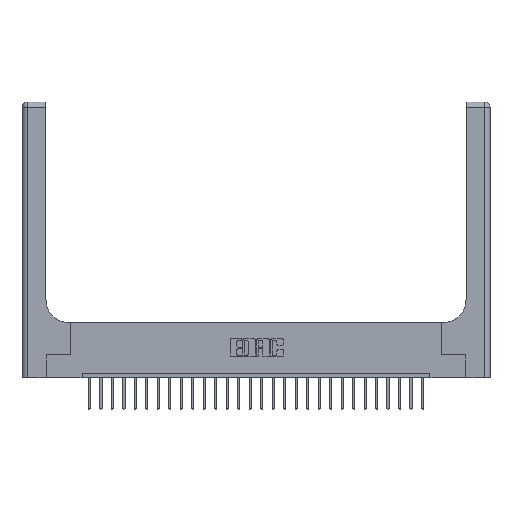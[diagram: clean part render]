
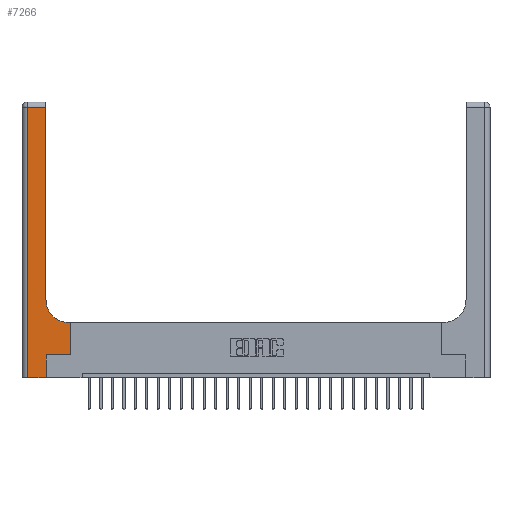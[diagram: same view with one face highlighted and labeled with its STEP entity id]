
A CAD part, top view. The second image highlights one B-rep face of the part: STEP entity #7266.
In plain terms, the highlighted planar face has unit normal (0, 0, 1).
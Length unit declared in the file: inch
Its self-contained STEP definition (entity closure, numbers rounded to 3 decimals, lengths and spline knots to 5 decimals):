
#961 = DIRECTION ( 'NONE',  ( 0., 1., 0. ) ) ;
#1334 = VECTOR ( 'NONE', #24281, 39.37008 ) ;
#1425 = EDGE_CURVE ( 'NONE', #2636, #16822, #12654, .T. ) ;
#1494 = DIRECTION ( 'NONE',  ( -1., 0., 0. ) ) ;
#1796 = CARTESIAN_POINT ( 'NONE',  ( 0.528, 0.6, 0.37 ) ) ;
#2108 = CARTESIAN_POINT ( 'NONE',  ( 0.265, 0., 0.37 ) ) ;
#2231 = CARTESIAN_POINT ( 'NONE',  ( 0., 0., 0.37 ) ) ;
#2236 = CARTESIAN_POINT ( 'NONE',  ( 0.26, 0.85, 0.37 ) ) ;
#2301 = VECTOR ( 'NONE', #20132, 39.37008 ) ;
#2636 = VERTEX_POINT ( 'NONE', #6936 ) ;
#2758 = VECTOR ( 'NONE', #10732, 39.37008 ) ;
#2800 = CARTESIAN_POINT ( 'NONE',  ( 0.06, 0., 0.37 ) ) ;
#2827 = CARTESIAN_POINT ( 'NONE',  ( 0.51, 0.6, 0.37 ) ) ;
#2962 = CARTESIAN_POINT ( 'NONE',  ( 0.528, 0.25, 0.37 ) ) ;
#3476 = CARTESIAN_POINT ( 'NONE',  ( 0., 3., 0.37 ) ) ;
#4074 = EDGE_CURVE ( 'NONE', #16822, #13934, #15352, .T. ) ;
#5895 = DIRECTION ( 'NONE',  ( -1., 0., 0. ) ) ;
#6661 = VERTEX_POINT ( 'NONE', #17787 ) ;
#6698 = VERTEX_POINT ( 'NONE', #2108 ) ;
#6707 = LINE ( 'NONE', #2231, #15286 ) ;
#6883 = CARTESIAN_POINT ( 'NONE',  ( 0.265, 0., 0.37 ) ) ;
#6888 = EDGE_CURVE ( 'NONE', #24734, #6661, #19367, .T. ) ;
#6936 = CARTESIAN_POINT ( 'NONE',  ( 0.265, 0.25, 0.37 ) ) ;
#7266 = ADVANCED_FACE ( 'NONE', ( #25118 ), #19017, .F. ) ;
#7838 = ORIENTED_EDGE ( 'NONE', *, *, #13670, .T. ) ;
#8047 = AXIS2_PLACEMENT_3D ( 'NONE', #11164, #24943, #13139 ) ;
#8358 = VERTEX_POINT ( 'NONE', #2236 ) ;
#8933 = EDGE_CURVE ( 'NONE', #13934, #12907, #24109, .T. ) ;
#9384 = ORIENTED_EDGE ( 'NONE', *, *, #17125, .T. ) ;
#9866 = ORIENTED_EDGE ( 'NONE', *, *, #15569, .T. ) ;
#10262 = CARTESIAN_POINT ( 'NONE',  ( 0.26, 3., 0.37 ) ) ;
#10732 = DIRECTION ( 'NONE',  ( 0., 1., 0. ) ) ;
#11164 = CARTESIAN_POINT ( 'NONE',  ( 0.51, 0.85, 0.37 ) ) ;
#11544 = DIRECTION ( 'NONE',  ( 1., 0., 0. ) ) ;
#11683 = ORIENTED_EDGE ( 'NONE', *, *, #1425, .T. ) ;
#12654 = LINE ( 'NONE', #21332, #20659 ) ;
#12907 = VERTEX_POINT ( 'NONE', #2827 ) ;
#13139 = DIRECTION ( 'NONE',  ( 1., 0., 0. ) ) ;
#13670 = EDGE_CURVE ( 'NONE', #23926, #6698, #6707, .T. ) ;
#13934 = VERTEX_POINT ( 'NONE', #1796 ) ;
#13953 = CARTESIAN_POINT ( 'NONE',  ( 0.26, 0.6, 0.37 ) ) ;
#14680 = ORIENTED_EDGE ( 'NONE', *, *, #4074, .T. ) ;
#15101 = CARTESIAN_POINT ( 'NONE',  ( 0.528, 0.25, 0.37 ) ) ;
#15286 = VECTOR ( 'NONE', #17718, 39.37008 ) ;
#15352 = LINE ( 'NONE', #2962, #2758 ) ;
#15569 = EDGE_CURVE ( 'NONE', #6661, #23926, #19903, .T. ) ;
#15830 = LINE ( 'NONE', #6883, #19542 ) ;
#16517 = AXIS2_PLACEMENT_3D ( 'NONE', #3476, #22923, #1494 ) ;
#16822 = VERTEX_POINT ( 'NONE', #15101 ) ;
#17125 = EDGE_CURVE ( 'NONE', #6698, #2636, #15830, .T. ) ;
#17254 = VECTOR ( 'NONE', #5895, 39.37008 ) ;
#17718 = DIRECTION ( 'NONE',  ( 1., 0., 0. ) ) ;
#17787 = CARTESIAN_POINT ( 'NONE',  ( 0.06, 2.94, 0.37 ) ) ;
#18195 = ORIENTED_EDGE ( 'NONE', *, *, #8933, .T. ) ;
#18357 = ORIENTED_EDGE ( 'NONE', *, *, #6888, .T. ) ;
#18408 = VECTOR ( 'NONE', #18830, 39.37008 ) ;
#18830 = DIRECTION ( 'NONE',  ( 0., -1., 0. ) ) ;
#19017 = PLANE ( 'NONE',  #16517 ) ;
#19100 = CARTESIAN_POINT ( 'NONE',  ( 0.26, 2.94, 0.37 ) ) ;
#19367 = LINE ( 'NONE', #21484, #17254 ) ;
#19542 = VECTOR ( 'NONE', #961, 39.37008 ) ;
#19903 = LINE ( 'NONE', #20697, #18408 ) ;
#20132 = DIRECTION ( 'NONE',  ( -1., 0., 0. ) ) ;
#20649 = CIRCLE ( 'NONE', #8047, 0.25 ) ;
#20659 = VECTOR ( 'NONE', #11544, 39.37008 ) ;
#20697 = CARTESIAN_POINT ( 'NONE',  ( 0.06, 3., 0.37 ) ) ;
#21332 = CARTESIAN_POINT ( 'NONE',  ( 0.265, 0.25, 0.37 ) ) ;
#21382 = ORIENTED_EDGE ( 'NONE', *, *, #24130, .T. ) ;
#21484 = CARTESIAN_POINT ( 'NONE',  ( 0., 2.94, 0.37 ) ) ;
#22812 = EDGE_LOOP ( 'NONE', ( #23235, #18357, #9866, #7838, #9384, #11683, #14680, #18195, #21382 ) ) ;
#22923 = DIRECTION ( 'NONE',  ( 0., 0., -1. ) ) ;
#23235 = ORIENTED_EDGE ( 'NONE', *, *, #23403, .T. ) ;
#23403 = EDGE_CURVE ( 'NONE', #8358, #24734, #23740, .T. ) ;
#23740 = LINE ( 'NONE', #10262, #1334 ) ;
#23926 = VERTEX_POINT ( 'NONE', #2800 ) ;
#24109 = LINE ( 'NONE', #13953, #2301 ) ;
#24130 = EDGE_CURVE ( 'NONE', #12907, #8358, #20649, .T. ) ;
#24281 = DIRECTION ( 'NONE',  ( 0., 1., 0. ) ) ;
#24734 = VERTEX_POINT ( 'NONE', #19100 ) ;
#24943 = DIRECTION ( 'NONE',  ( 0., 0., -1. ) ) ;
#25118 = FACE_OUTER_BOUND ( 'NONE', #22812, .T. ) ;
